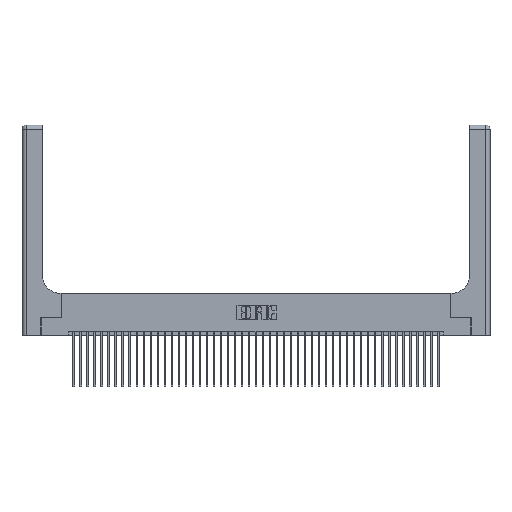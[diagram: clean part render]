
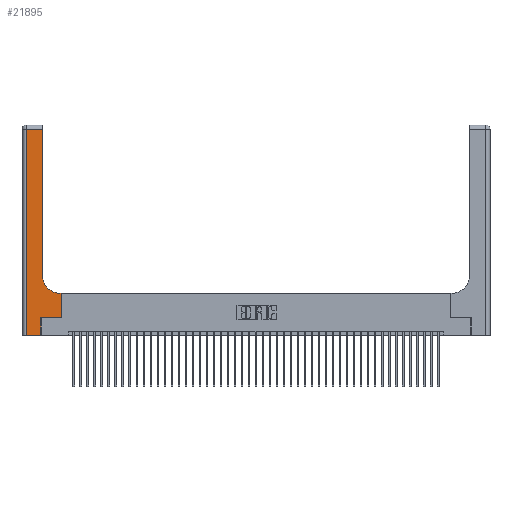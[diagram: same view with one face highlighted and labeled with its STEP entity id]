
A CAD part, top view. The second image highlights one B-rep face of the part: STEP entity #21895.
In plain terms, the highlighted planar face has unit normal (0, 0, 1).
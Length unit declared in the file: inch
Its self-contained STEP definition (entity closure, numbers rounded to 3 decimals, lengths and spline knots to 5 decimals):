
#498 = LINE ( 'NONE', #32065, #8774 ) ;
#572 = EDGE_CURVE ( 'NONE', #43254, #8964, #16661, .T. ) ;
#933 = ORIENTED_EDGE ( 'NONE', *, *, #572, .T. ) ;
#1397 = VERTEX_POINT ( 'NONE', #30245 ) ;
#1502 = VECTOR ( 'NONE', #13533, 39.37008 ) ;
#1615 = LINE ( 'NONE', #41927, #20322 ) ;
#1748 = AXIS2_PLACEMENT_3D ( 'NONE', #3873, #28417, #7414 ) ;
#2925 = CARTESIAN_POINT ( 'NONE',  ( 0.06, 0., 0.37 ) ) ;
#3159 = CARTESIAN_POINT ( 'NONE',  ( 0.5585, 0.25, 0.37 ) ) ;
#3318 = VERTEX_POINT ( 'NONE', #36933 ) ;
#3861 = LINE ( 'NONE', #12582, #40036 ) ;
#3873 = CARTESIAN_POINT ( 'NONE',  ( 0.5415, 0.85, 0.37 ) ) ;
#4756 = CARTESIAN_POINT ( 'NONE',  ( 0.269, 0.25, 0.37 ) ) ;
#4776 = ORIENTED_EDGE ( 'NONE', *, *, #45045, .T. ) ;
#5378 = DIRECTION ( 'NONE',  ( 1., 0., 0. ) ) ;
#6318 = EDGE_CURVE ( 'NONE', #24071, #3318, #44446, .T. ) ;
#6610 = VERTEX_POINT ( 'NONE', #24547 ) ;
#6832 = EDGE_CURVE ( 'NONE', #3318, #26680, #43933, .T. ) ;
#7414 = DIRECTION ( 'NONE',  ( 1., 0., 0. ) ) ;
#7891 = VERTEX_POINT ( 'NONE', #18154 ) ;
#8123 = EDGE_CURVE ( 'NONE', #33595, #7891, #1615, .T. ) ;
#8279 = CIRCLE ( 'NONE', #1748, 0.25 ) ;
#8326 = FACE_OUTER_BOUND ( 'NONE', #8432, .T. ) ;
#8432 = EDGE_LOOP ( 'NONE', ( #20184, #22374, #4776, #14171, #34951, #27839, #933, #13635, #32260 ) ) ;
#8774 = VECTOR ( 'NONE', #35552, 39.37008 ) ;
#8964 = VERTEX_POINT ( 'NONE', #25833 ) ;
#10752 = CARTESIAN_POINT ( 'NONE',  ( 0., 3., 0.37 ) ) ;
#11495 = DIRECTION ( 'NONE',  ( 0., 1., 0. ) ) ;
#12582 = CARTESIAN_POINT ( 'NONE',  ( 0.269, 0.25, 0.37 ) ) ;
#13533 = DIRECTION ( 'NONE',  ( 0., -1., 0. ) ) ;
#13635 = ORIENTED_EDGE ( 'NONE', *, *, #27605, .T. ) ;
#14171 = ORIENTED_EDGE ( 'NONE', *, *, #6318, .T. ) ;
#14282 = DIRECTION ( 'NONE',  ( 0., 0., -1. ) ) ;
#15712 = CARTESIAN_POINT ( 'NONE',  ( 0.2915, 2.94, 0.37 ) ) ;
#16661 = LINE ( 'NONE', #21902, #34185 ) ;
#17485 = DIRECTION ( 'NONE',  ( -1., 0., 0. ) ) ;
#18154 = CARTESIAN_POINT ( 'NONE',  ( 0.06, 2.94, 0.37 ) ) ;
#18629 = AXIS2_PLACEMENT_3D ( 'NONE', #10752, #14282, #38712 ) ;
#19610 = DIRECTION ( 'NONE',  ( 1., 0., 0. ) ) ;
#20184 = ORIENTED_EDGE ( 'NONE', *, *, #34050, .T. ) ;
#20322 = VECTOR ( 'NONE', #17485, 39.37008 ) ;
#21895 = ADVANCED_FACE ( 'NONE', ( #8326 ), #31722, .F. ) ;
#21902 = CARTESIAN_POINT ( 'NONE',  ( 0.5585, 0.25, 0.37 ) ) ;
#22374 = ORIENTED_EDGE ( 'NONE', *, *, #8123, .T. ) ;
#24071 = VERTEX_POINT ( 'NONE', #2925 ) ;
#24547 = CARTESIAN_POINT ( 'NONE',  ( 0.5415, 0.6, 0.37 ) ) ;
#25833 = CARTESIAN_POINT ( 'NONE',  ( 0.5585, 0.6, 0.37 ) ) ;
#25879 = VECTOR ( 'NONE', #5378, 39.37008 ) ;
#26680 = VERTEX_POINT ( 'NONE', #4756 ) ;
#27083 = DIRECTION ( 'NONE',  ( -1., 0., 0. ) ) ;
#27465 = LINE ( 'NONE', #44489, #44931 ) ;
#27517 = EDGE_CURVE ( 'NONE', #26680, #43254, #3861, .T. ) ;
#27605 = EDGE_CURVE ( 'NONE', #8964, #6610, #27465, .T. ) ;
#27839 = ORIENTED_EDGE ( 'NONE', *, *, #27517, .T. ) ;
#28417 = DIRECTION ( 'NONE',  ( 0., 0., -1. ) ) ;
#30245 = CARTESIAN_POINT ( 'NONE',  ( 0.2915, 0.85, 0.37 ) ) ;
#30975 = CARTESIAN_POINT ( 'NONE',  ( 0.06, 3., 0.37 ) ) ;
#31722 = PLANE ( 'NONE',  #18629 ) ;
#32065 = CARTESIAN_POINT ( 'NONE',  ( 0.2915, 3., 0.37 ) ) ;
#32260 = ORIENTED_EDGE ( 'NONE', *, *, #33383, .T. ) ;
#33116 = CARTESIAN_POINT ( 'NONE',  ( 0.269, 0., 0.37 ) ) ;
#33383 = EDGE_CURVE ( 'NONE', #6610, #1397, #8279, .T. ) ;
#33595 = VERTEX_POINT ( 'NONE', #15712 ) ;
#34050 = EDGE_CURVE ( 'NONE', #1397, #33595, #498, .T. ) ;
#34185 = VECTOR ( 'NONE', #11495, 39.37008 ) ;
#34951 = ORIENTED_EDGE ( 'NONE', *, *, #6832, .T. ) ;
#35552 = DIRECTION ( 'NONE',  ( 0., 1., 0. ) ) ;
#36587 = DIRECTION ( 'NONE',  ( 0., 1., 0. ) ) ;
#36933 = CARTESIAN_POINT ( 'NONE',  ( 0.269, 0., 0.37 ) ) ;
#38712 = DIRECTION ( 'NONE',  ( -1., 0., 0. ) ) ;
#38779 = LINE ( 'NONE', #30975, #1502 ) ;
#40036 = VECTOR ( 'NONE', #19610, 39.37008 ) ;
#40295 = CARTESIAN_POINT ( 'NONE',  ( 0., 0., 0.37 ) ) ;
#41927 = CARTESIAN_POINT ( 'NONE',  ( 0., 2.94, 0.37 ) ) ;
#42819 = VECTOR ( 'NONE', #36587, 39.37008 ) ;
#43254 = VERTEX_POINT ( 'NONE', #3159 ) ;
#43933 = LINE ( 'NONE', #33116, #42819 ) ;
#44446 = LINE ( 'NONE', #40295, #25879 ) ;
#44489 = CARTESIAN_POINT ( 'NONE',  ( 0.2915, 0.6, 0.37 ) ) ;
#44931 = VECTOR ( 'NONE', #27083, 39.37008 ) ;
#45045 = EDGE_CURVE ( 'NONE', #7891, #24071, #38779, .T. ) ;
